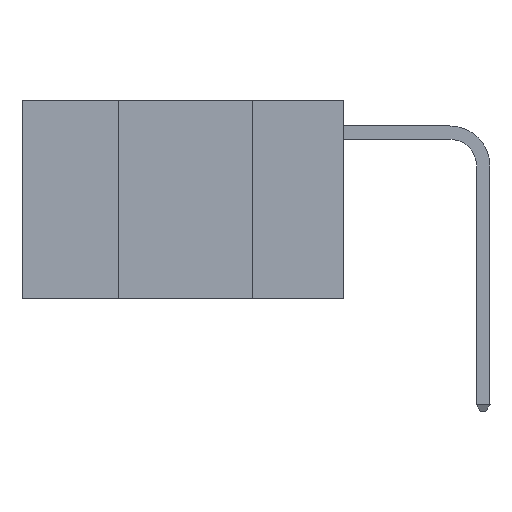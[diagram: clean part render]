
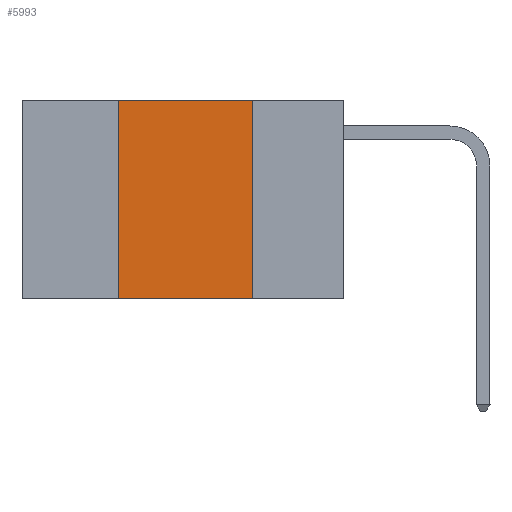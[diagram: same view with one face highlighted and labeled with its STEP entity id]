
A CAD part, left-side view. The second image highlights one B-rep face of the part: STEP entity #5993.
In plain terms, the highlighted planar face has unit normal (-1, 0, 0).
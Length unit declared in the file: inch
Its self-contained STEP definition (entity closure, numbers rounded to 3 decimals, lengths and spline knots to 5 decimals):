
#922 = CARTESIAN_POINT ( 'NONE',  ( 0., 0.42, 0. ) ) ;
#1237 = VECTOR ( 'NONE', #2662, 39.37008 ) ;
#1642 = EDGE_CURVE ( 'NONE', #8952, #7030, #5251, .T. ) ;
#1842 = CARTESIAN_POINT ( 'NONE',  ( 0., 0.6, -0.37 ) ) ;
#2662 = DIRECTION ( 'NONE',  ( 0., -1., 0. ) ) ;
#2758 = LINE ( 'NONE', #4264, #1237 ) ;
#3001 = VECTOR ( 'NONE', #3903, 39.37008 ) ;
#3166 = CARTESIAN_POINT ( 'NONE',  ( 0., 0.17, 0. ) ) ;
#3229 = CARTESIAN_POINT ( 'NONE',  ( 0., 0.42, 0. ) ) ;
#3444 = ORIENTED_EDGE ( 'NONE', *, *, #8133, .F. ) ;
#3581 = VECTOR ( 'NONE', #4040, 39.37008 ) ;
#3657 = DIRECTION ( 'NONE',  ( 1., 0., 0. ) ) ;
#3746 = AXIS2_PLACEMENT_3D ( 'NONE', #7563, #3657, #8306 ) ;
#3903 = DIRECTION ( 'NONE',  ( 0., 0., 1. ) ) ;
#4040 = DIRECTION ( 'NONE',  ( 0., -1., 0. ) ) ;
#4264 = CARTESIAN_POINT ( 'NONE',  ( 0., 0.6, 0. ) ) ;
#4498 = FACE_OUTER_BOUND ( 'NONE', #5701, .T. ) ;
#4546 = PLANE ( 'NONE',  #3746 ) ;
#5251 = LINE ( 'NONE', #922, #3001 ) ;
#5419 = LINE ( 'NONE', #3166, #6272 ) ;
#5433 = CARTESIAN_POINT ( 'NONE',  ( 0., 0.17, 0. ) ) ;
#5586 = ORIENTED_EDGE ( 'NONE', *, *, #8442, .T. ) ;
#5701 = EDGE_LOOP ( 'NONE', ( #8149, #3444, #8951, #5586 ) ) ;
#5844 = VERTEX_POINT ( 'NONE', #5433 ) ;
#5993 = ADVANCED_FACE ( 'NONE', ( #4498 ), #4546, .F. ) ;
#6024 = VERTEX_POINT ( 'NONE', #6814 ) ;
#6176 = DIRECTION ( 'NONE',  ( 0., 0., -1. ) ) ;
#6272 = VECTOR ( 'NONE', #6176, 39.37008 ) ;
#6412 = CARTESIAN_POINT ( 'NONE',  ( 0., 0.42, -0.37 ) ) ;
#6814 = CARTESIAN_POINT ( 'NONE',  ( 0., 0.17, -0.37 ) ) ;
#7030 = VERTEX_POINT ( 'NONE', #3229 ) ;
#7563 = CARTESIAN_POINT ( 'NONE',  ( 0., 0.6, 0. ) ) ;
#7806 = LINE ( 'NONE', #1842, #3581 ) ;
#8133 = EDGE_CURVE ( 'NONE', #7030, #5844, #2758, .T. ) ;
#8149 = ORIENTED_EDGE ( 'NONE', *, *, #8512, .F. ) ;
#8306 = DIRECTION ( 'NONE',  ( 0., 0., -1. ) ) ;
#8442 = EDGE_CURVE ( 'NONE', #8952, #6024, #7806, .T. ) ;
#8512 = EDGE_CURVE ( 'NONE', #5844, #6024, #5419, .T. ) ;
#8951 = ORIENTED_EDGE ( 'NONE', *, *, #1642, .F. ) ;
#8952 = VERTEX_POINT ( 'NONE', #6412 ) ;
